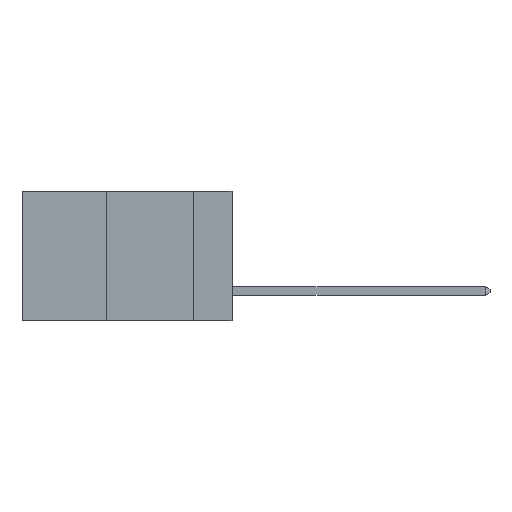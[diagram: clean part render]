
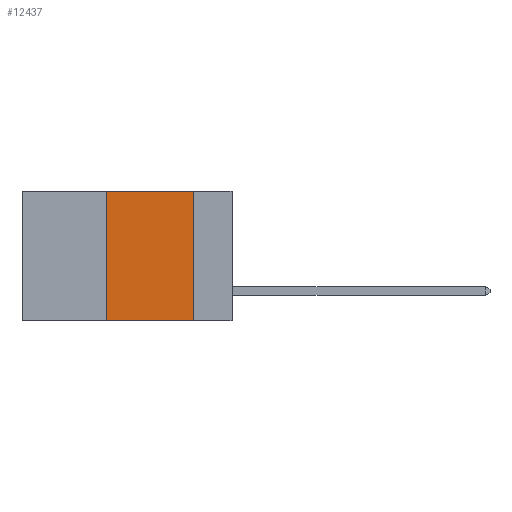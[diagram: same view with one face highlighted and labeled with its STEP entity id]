
A CAD part, left-side view. The second image highlights one B-rep face of the part: STEP entity #12437.
In plain terms, the highlighted planar face has unit normal (-1, 0, 0).
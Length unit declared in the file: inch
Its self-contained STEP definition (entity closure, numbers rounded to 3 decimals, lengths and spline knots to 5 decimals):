
#885 = CARTESIAN_POINT ( 'NONE',  ( 0., 0.36, 0. ) ) ;
#1797 = CARTESIAN_POINT ( 'NONE',  ( 0., 0.36, -0.37 ) ) ;
#2324 = VERTEX_POINT ( 'NONE', #3086 ) ;
#3086 = CARTESIAN_POINT ( 'NONE',  ( 0., 0.11, -0.37 ) ) ;
#3314 = DIRECTION ( 'NONE',  ( 0., 0., -1. ) ) ;
#3803 = VECTOR ( 'NONE', #28524, 39.37008 ) ;
#3948 = EDGE_CURVE ( 'NONE', #5448, #24995, #18836, .T. ) ;
#5062 = VERTEX_POINT ( 'NONE', #1797 ) ;
#5448 = VERTEX_POINT ( 'NONE', #885 ) ;
#5692 = VECTOR ( 'NONE', #13806, 39.37008 ) ;
#8164 = DIRECTION ( 'NONE',  ( 0., -1., 0. ) ) ;
#8746 = AXIS2_PLACEMENT_3D ( 'NONE', #14502, #16773, #3314 ) ;
#9981 = VECTOR ( 'NONE', #8164, 39.37008 ) ;
#10423 = ORIENTED_EDGE ( 'NONE', *, *, #22025, .F. ) ;
#10601 = ORIENTED_EDGE ( 'NONE', *, *, #3948, .F. ) ;
#10722 = ORIENTED_EDGE ( 'NONE', *, *, #26854, .F. ) ;
#10887 = ORIENTED_EDGE ( 'NONE', *, *, #25419, .T. ) ;
#12437 = ADVANCED_FACE ( 'NONE', ( #22639 ), #27542, .F. ) ;
#12879 = VECTOR ( 'NONE', #22432, 39.37008 ) ;
#13308 = CARTESIAN_POINT ( 'NONE',  ( 0., 0.11, 0. ) ) ;
#13806 = DIRECTION ( 'NONE',  ( 0., 0., 1. ) ) ;
#14502 = CARTESIAN_POINT ( 'NONE',  ( 0., 0.6, 0. ) ) ;
#15725 = LINE ( 'NONE', #13308, #3803 ) ;
#16773 = DIRECTION ( 'NONE',  ( 1., 0., 0. ) ) ;
#17816 = CARTESIAN_POINT ( 'NONE',  ( 0., 0.11, 0. ) ) ;
#18836 = LINE ( 'NONE', #20261, #12879 ) ;
#19305 = CARTESIAN_POINT ( 'NONE',  ( 0., 0.6, -0.37 ) ) ;
#20261 = CARTESIAN_POINT ( 'NONE',  ( 0., 0.6, 0. ) ) ;
#21779 = LINE ( 'NONE', #19305, #9981 ) ;
#22025 = EDGE_CURVE ( 'NONE', #24995, #2324, #15725, .T. ) ;
#22086 = EDGE_LOOP ( 'NONE', ( #10423, #10601, #10722, #10887 ) ) ;
#22432 = DIRECTION ( 'NONE',  ( 0., -1., 0. ) ) ;
#22639 = FACE_OUTER_BOUND ( 'NONE', #22086, .T. ) ;
#22713 = LINE ( 'NONE', #26891, #5692 ) ;
#24995 = VERTEX_POINT ( 'NONE', #17816 ) ;
#25419 = EDGE_CURVE ( 'NONE', #5062, #2324, #21779, .T. ) ;
#26854 = EDGE_CURVE ( 'NONE', #5062, #5448, #22713, .T. ) ;
#26891 = CARTESIAN_POINT ( 'NONE',  ( 0., 0.36, 0. ) ) ;
#27542 = PLANE ( 'NONE',  #8746 ) ;
#28524 = DIRECTION ( 'NONE',  ( 0., 0., -1. ) ) ;
